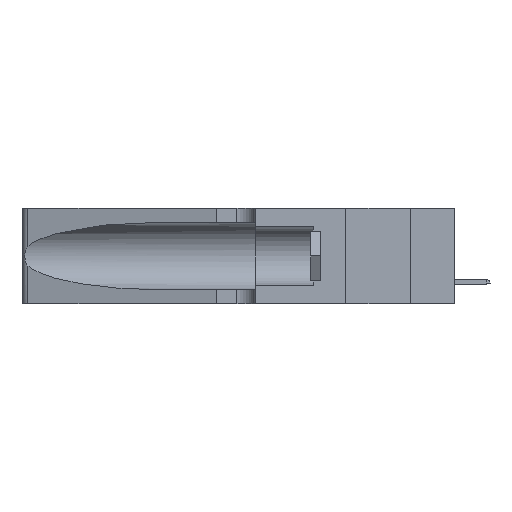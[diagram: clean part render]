
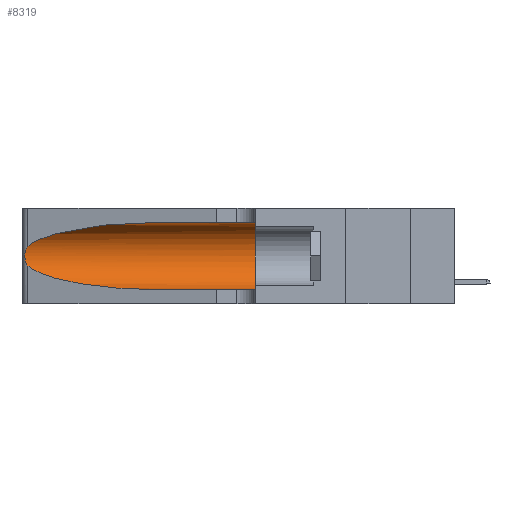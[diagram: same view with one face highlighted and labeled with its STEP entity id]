
A CAD part, left-side view. The second image highlights one B-rep face of the part: STEP entity #8319.
In plain terms, the highlighted cylindrical face has radius 3.308 mm (diameter 6.617 mm), a partial arc.
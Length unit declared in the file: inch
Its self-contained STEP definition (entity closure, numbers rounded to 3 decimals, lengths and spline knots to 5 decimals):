
#745 = FACE_OUTER_BOUND ( 'NONE', #1831, .T. ) ;
#1039 = EDGE_CURVE ( 'NONE', #50677, #27804, #41892, .T. ) ;
#1831 = EDGE_LOOP ( 'NONE', ( #45662, #5904, #18379, #8629, #27817, #21469 ) ) ;
#2547 = CARTESIAN_POINT ( 'NONE',  ( 0.1305, 0.35, 0.185 ) ) ;
#3028 = CARTESIAN_POINT ( 'NONE',  ( 0.25856, 1.23593, 0.16098 ) ) ;
#3282 = CARTESIAN_POINT ( 'NONE',  ( 0.25555, 1.22993, 0.14849 ) ) ;
#3534 = CARTESIAN_POINT ( 'NONE',  ( 0.26018, 1.23835, 0.19895 ) ) ;
#3754 = VECTOR ( 'NONE', #41627, 39.37008 ) ;
#3903 = CARTESIAN_POINT ( 'NONE',  ( 0.25487, 1.22718, 0.14631 ) ) ;
#4264 = VERTEX_POINT ( 'NONE', #36860 ) ;
#5673 = CARTESIAN_POINT ( 'NONE',  ( 0.25487, 1.22718, 0.22369 ) ) ;
#5904 = ORIENTED_EDGE ( 'NONE', *, *, #26385, .T. ) ;
#6417 = DIRECTION ( 'NONE',  ( 0., 0., 1. ) ) ;
#7096 = AXIS2_PLACEMENT_3D ( 'NONE', #2547, #46880, #6417 ) ;
#7796 =( BOUNDED_CURVE ( )  B_SPLINE_CURVE ( 3, ( #29305, #9575, #41236, #5673 ),
 .UNSPECIFIED., .F., .T. ) 
 B_SPLINE_CURVE_WITH_KNOTS ( ( 4, 4 ),
 ( 1.5708, 2.84003 ),
 .UNSPECIFIED. ) 
 CURVE ( )  GEOMETRIC_REPRESENTATION_ITEM ( )  RATIONAL_B_SPLINE_CURVE ( ( 1., 0.87, 0.87, 1. ) ) 
 REPRESENTATION_ITEM ( '' )  );
#8033 = DIRECTION ( 'NONE',  ( 0., -1., 0. ) ) ;
#8319 = ADVANCED_FACE ( 'NONE', ( #745 ), #15830, .F. ) ;
#8523 = EDGE_CURVE ( 'NONE', #24573, #15186, #7796, .T. ) ;
#8629 = ORIENTED_EDGE ( 'NONE', *, *, #38024, .T. ) ;
#9575 = CARTESIAN_POINT ( 'NONE',  ( 0.18966, 0.96281, 0.31525 ) ) ;
#9583 = CARTESIAN_POINT ( 'NONE',  ( 0.25487, 1.22718, 0.22369 ) ) ;
#11311 = CARTESIAN_POINT ( 'NONE',  ( 0.26017, 1.23833, 0.17102 ) ) ;
#15119 = CARTESIAN_POINT ( 'NONE',  ( 0.1305, 0.35, 0.31525 ) ) ;
#15186 = VERTEX_POINT ( 'NONE', #9583 ) ;
#15208 = CARTESIAN_POINT ( 'NONE',  ( 0.25555, 1.22994, 0.2215 ) ) ;
#15830 = CYLINDRICAL_SURFACE ( 'NONE', #24853, 0.13025 ) ;
#17799 = LINE ( 'NONE', #33908, #46384 ) ;
#18379 = ORIENTED_EDGE ( 'NONE', *, *, #25409, .T. ) ;
#19025 = CARTESIAN_POINT ( 'NONE',  ( 0.1305, 0.35, 0.05475 ) ) ;
#20474 = DIRECTION ( 'NONE',  ( 0., 0., -1. ) ) ;
#20854 = LINE ( 'NONE', #29156, #3754 ) ;
#21469 = ORIENTED_EDGE ( 'NONE', *, *, #28319, .F. ) ;
#22298 = VERTEX_POINT ( 'NONE', #3903 ) ;
#22494 = CARTESIAN_POINT ( 'NONE',  ( 0.25639, 1.23184, 0.21858 ) ) ;
#24031 =( BOUNDED_CURVE ( )  B_SPLINE_CURVE ( 3, ( #41843, #34047, #49855, #37147 ),
 .UNSPECIFIED., .F., .T. ) 
 B_SPLINE_CURVE_WITH_KNOTS ( ( 4, 4 ),
 ( 3.44316, 4.71239 ),
 .UNSPECIFIED. ) 
 CURVE ( )  GEOMETRIC_REPRESENTATION_ITEM ( )  RATIONAL_B_SPLINE_CURVE ( ( 1., 0.87, 0.87, 1. ) ) 
 REPRESENTATION_ITEM ( '' )  );
#24573 = VERTEX_POINT ( 'NONE', #44854 ) ;
#24853 = AXIS2_PLACEMENT_3D ( 'NONE', #48486, #8033, #20474 ) ;
#25409 = EDGE_CURVE ( 'NONE', #22298, #4264, #24031, .T. ) ;
#26138 = CARTESIAN_POINT ( 'NONE',  ( 0.25487, 1.22718, 0.22369 ) ) ;
#26385 = EDGE_CURVE ( 'NONE', #15186, #22298, #48017, .T. ) ;
#27148 = CARTESIAN_POINT ( 'NONE',  ( 0.25639, 1.23186, 0.15144 ) ) ;
#27804 = VERTEX_POINT ( 'NONE', #19025 ) ;
#27817 = ORIENTED_EDGE ( 'NONE', *, *, #1039, .F. ) ;
#28319 = EDGE_CURVE ( 'NONE', #24573, #50677, #20854, .T. ) ;
#29156 = CARTESIAN_POINT ( 'NONE',  ( 0.1305, 1.61858, 0.31525 ) ) ;
#29305 = CARTESIAN_POINT ( 'NONE',  ( 0.1305, 0.72297, 0.31525 ) ) ;
#33649 = DIRECTION ( 'NONE',  ( 0., -1., 0. ) ) ;
#33908 = CARTESIAN_POINT ( 'NONE',  ( 0.1305, 1.61858, 0.05475 ) ) ;
#34047 = CARTESIAN_POINT ( 'NONE',  ( 0.2373, 1.15595, 0.08982 ) ) ;
#36860 = CARTESIAN_POINT ( 'NONE',  ( 0.1305, 0.72297, 0.05475 ) ) ;
#37147 = CARTESIAN_POINT ( 'NONE',  ( 0.1305, 0.72297, 0.05475 ) ) ;
#38024 = EDGE_CURVE ( 'NONE', #4264, #27804, #17799, .T. ) ;
#38057 = CARTESIAN_POINT ( 'NONE',  ( 0.26075, 1.23896, 0.19203 ) ) ;
#41236 = CARTESIAN_POINT ( 'NONE',  ( 0.2373, 1.15595, 0.28018 ) ) ;
#41627 = DIRECTION ( 'NONE',  ( 0., -1., 0. ) ) ;
#41843 = CARTESIAN_POINT ( 'NONE',  ( 0.25487, 1.22718, 0.14631 ) ) ;
#41892 = CIRCLE ( 'NONE', #7096, 0.13025 ) ;
#42230 = CARTESIAN_POINT ( 'NONE',  ( 0.26075, 1.23896, 0.178 ) ) ;
#42490 = CARTESIAN_POINT ( 'NONE',  ( 0.25854, 1.2359, 0.20912 ) ) ;
#44854 = CARTESIAN_POINT ( 'NONE',  ( 0.1305, 0.72297, 0.31525 ) ) ;
#45662 = ORIENTED_EDGE ( 'NONE', *, *, #8523, .T. ) ;
#46384 = VECTOR ( 'NONE', #33649, 39.37008 ) ;
#46842 = CARTESIAN_POINT ( 'NONE',  ( 0.25787, 1.23484, 0.2124 ) ) ;
#46880 = DIRECTION ( 'NONE',  ( 0., 1., 0. ) ) ;
#48017 = B_SPLINE_CURVE_WITH_KNOTS ( 'NONE', 3,
 ( #26138, #15208, #22494, #46842, #42490, #3534, #38057, #42230, #11311, #3028, #50490, #27148, #3282, #49987 ),
 .UNSPECIFIED., .F., .F.,
 ( 4, 2, 2, 2, 2, 2, 4 ),
 ( 0., 0.00027, 0.00053, 0.00107, 0.0016, 0.00187, 0.00214 ),
 .UNSPECIFIED. ) ;
#48486 = CARTESIAN_POINT ( 'NONE',  ( 0.1305, 1.61858, 0.185 ) ) ;
#49855 = CARTESIAN_POINT ( 'NONE',  ( 0.18966, 0.96281, 0.05475 ) ) ;
#49987 = CARTESIAN_POINT ( 'NONE',  ( 0.25487, 1.22718, 0.14631 ) ) ;
#50490 = CARTESIAN_POINT ( 'NONE',  ( 0.25789, 1.23486, 0.15765 ) ) ;
#50677 = VERTEX_POINT ( 'NONE', #15119 ) ;
